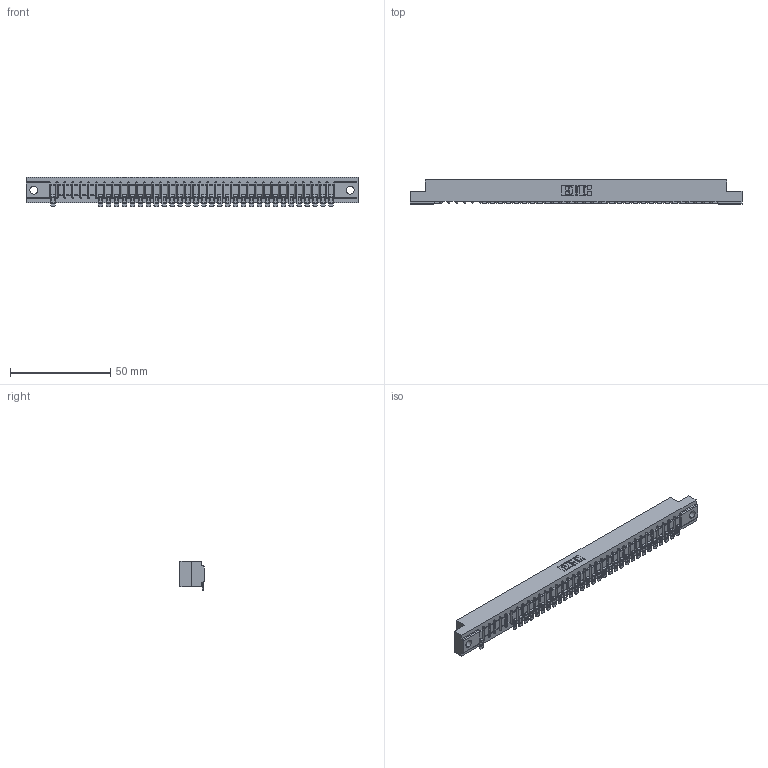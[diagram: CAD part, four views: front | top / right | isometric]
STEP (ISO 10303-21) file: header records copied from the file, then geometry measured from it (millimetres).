
FILE_DESCRIPTION (( 'STEP AP203' ), '1' );
FILE_NAME ('357-036-554-104.STEP', '2018-08-10T05:56:29', ( '' ), ( '' ), 'SwSTEP 2.0', 'SolidWorks 2016', '' );
FILE_SCHEMA (( 'CONFIG_CONTROL_DESIGN' ));
Length unit declared in the file: inch
Products named in the file (3): 307 Part_.156 Dia Mounting Holes; 307-290-002_554; 357-036-554-104
Assembly tree (32 placements, depth 2):
  357-036-554-104
    307 Part_.156 Dia Mounting Holes
    307-290-002_554  x31
Bounding box: 165.66 x 12.01 x 14.52 mm (x, y, z)
Volume: 17443.4 mm3; surface area: 20829.7 mm2
Topology: 32 solids, 32 shells, 2780 faces, 8522 edges, 5580 vertices
Faces by surface type: plane 1570, cylinder 1136, sphere 74
Entity records: 32825 total; most frequent: CARTESIAN_POINT 5563, ORIENTED_EDGE 5556, DIRECTION 5400, EDGE_CURVE 2778, LINE 2126, VECTOR 2126, VERTEX_POINT 1800, AXIS2_PLACEMENT_3D 1637
